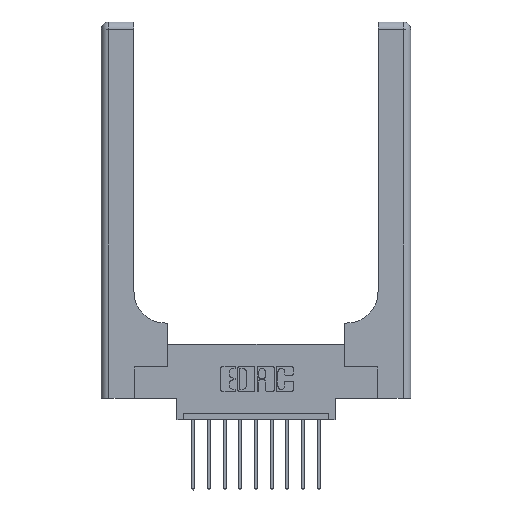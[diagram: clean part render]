
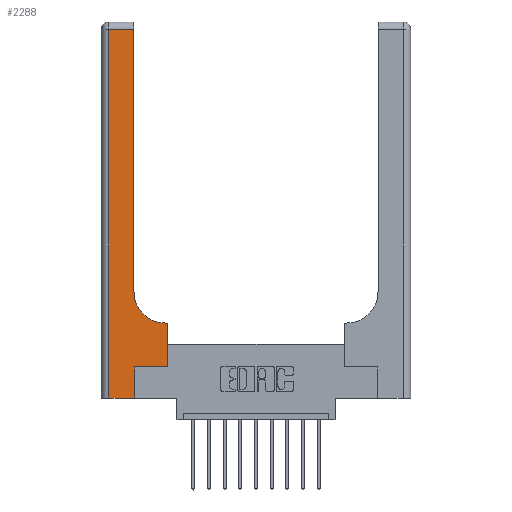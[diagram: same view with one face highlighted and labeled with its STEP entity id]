
A CAD part, top view. The second image highlights one B-rep face of the part: STEP entity #2288.
In plain terms, the highlighted planar face has unit normal (0, 0, 1).
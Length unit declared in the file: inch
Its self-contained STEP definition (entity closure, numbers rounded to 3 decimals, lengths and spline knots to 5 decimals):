
#54 = CARTESIAN_POINT ( 'NONE',  ( 0.51, 0.85, 0.37 ) ) ;
#245 = CARTESIAN_POINT ( 'NONE',  ( 0., 3., 0.37 ) ) ;
#322 = DIRECTION ( 'NONE',  ( 0., 1., 0. ) ) ;
#487 = VECTOR ( 'NONE', #4589, 39.37008 ) ;
#913 = ORIENTED_EDGE ( 'NONE', *, *, #4546, .T. ) ;
#1056 = VECTOR ( 'NONE', #8167, 39.37008 ) ;
#1525 = ORIENTED_EDGE ( 'NONE', *, *, #4933, .T. ) ;
#1647 = DIRECTION ( 'NONE',  ( 0., 1., 0. ) ) ;
#1715 = EDGE_LOOP ( 'NONE', ( #7475, #12008, #1525, #6539, #4272, #3460, #15296, #10799, #913 ) ) ;
#1851 = LINE ( 'NONE', #4492, #487 ) ;
#2288 = ADVANCED_FACE ( 'NONE', ( #4035 ), #2567, .F. ) ;
#2551 = EDGE_CURVE ( 'NONE', #13347, #2788, #5854, .T. ) ;
#2567 = PLANE ( 'NONE',  #7555 ) ;
#2635 = DIRECTION ( 'NONE',  ( 1., 0., 0. ) ) ;
#2788 = VERTEX_POINT ( 'NONE', #5135 ) ;
#3329 = EDGE_CURVE ( 'NONE', #9762, #10007, #15125, .T. ) ;
#3349 = CARTESIAN_POINT ( 'NONE',  ( 0.06, 0., 0.37 ) ) ;
#3460 = ORIENTED_EDGE ( 'NONE', *, *, #6564, .T. ) ;
#4035 = FACE_OUTER_BOUND ( 'NONE', #1715, .T. ) ;
#4132 = DIRECTION ( 'NONE',  ( -1., 0., 0. ) ) ;
#4255 = LINE ( 'NONE', #5275, #13698 ) ;
#4272 = ORIENTED_EDGE ( 'NONE', *, *, #3329, .T. ) ;
#4292 = VECTOR ( 'NONE', #4132, 39.37008 ) ;
#4322 = LINE ( 'NONE', #13469, #12302 ) ;
#4492 = CARTESIAN_POINT ( 'NONE',  ( 0.26, 0.6, 0.37 ) ) ;
#4546 = EDGE_CURVE ( 'NONE', #13623, #13347, #5232, .T. ) ;
#4589 = DIRECTION ( 'NONE',  ( -1., 0., 0. ) ) ;
#4761 = CARTESIAN_POINT ( 'NONE',  ( 0.26, 0.85, 0.37 ) ) ;
#4933 = EDGE_CURVE ( 'NONE', #6191, #13693, #4322, .T. ) ;
#5135 = CARTESIAN_POINT ( 'NONE',  ( 0.26, 2.94, 0.37 ) ) ;
#5178 = AXIS2_PLACEMENT_3D ( 'NONE', #54, #6262, #6154 ) ;
#5232 = CIRCLE ( 'NONE', #5178, 0.25 ) ;
#5275 = CARTESIAN_POINT ( 'NONE',  ( 0., 0., 0.37 ) ) ;
#5380 = LINE ( 'NONE', #6357, #12465 ) ;
#5854 = LINE ( 'NONE', #12187, #1056 ) ;
#6154 = DIRECTION ( 'NONE',  ( 1., 0., 0. ) ) ;
#6191 = VERTEX_POINT ( 'NONE', #14523 ) ;
#6262 = DIRECTION ( 'NONE',  ( 0., 0., -1. ) ) ;
#6357 = CARTESIAN_POINT ( 'NONE',  ( 0.265, 0.25, 0.37 ) ) ;
#6539 = ORIENTED_EDGE ( 'NONE', *, *, #7841, .T. ) ;
#6564 = EDGE_CURVE ( 'NONE', #10007, #10224, #5380, .T. ) ;
#7475 = ORIENTED_EDGE ( 'NONE', *, *, #2551, .T. ) ;
#7555 = AXIS2_PLACEMENT_3D ( 'NONE', #245, #13413, #12134 ) ;
#7587 = CARTESIAN_POINT ( 'NONE',  ( 0.528, 0.6, 0.37 ) ) ;
#7841 = EDGE_CURVE ( 'NONE', #13693, #9762, #4255, .T. ) ;
#8033 = CARTESIAN_POINT ( 'NONE',  ( 0.265, 0., 0.37 ) ) ;
#8057 = VECTOR ( 'NONE', #322, 39.37008 ) ;
#8167 = DIRECTION ( 'NONE',  ( 0., 1., 0. ) ) ;
#8651 = VECTOR ( 'NONE', #1647, 39.37008 ) ;
#8836 = DIRECTION ( 'NONE',  ( 0., -1., 0. ) ) ;
#9002 = CARTESIAN_POINT ( 'NONE',  ( 0.528, 0.25, 0.37 ) ) ;
#9458 = VERTEX_POINT ( 'NONE', #7587 ) ;
#9762 = VERTEX_POINT ( 'NONE', #8033 ) ;
#10007 = VERTEX_POINT ( 'NONE', #13125 ) ;
#10091 = EDGE_CURVE ( 'NONE', #10224, #9458, #12200, .T. ) ;
#10224 = VERTEX_POINT ( 'NONE', #9002 ) ;
#10799 = ORIENTED_EDGE ( 'NONE', *, *, #14190, .T. ) ;
#12008 = ORIENTED_EDGE ( 'NONE', *, *, #14170, .T. ) ;
#12134 = DIRECTION ( 'NONE',  ( -1., 0., 0. ) ) ;
#12187 = CARTESIAN_POINT ( 'NONE',  ( 0.26, 3., 0.37 ) ) ;
#12200 = LINE ( 'NONE', #12400, #8651 ) ;
#12302 = VECTOR ( 'NONE', #8836, 39.37008 ) ;
#12400 = CARTESIAN_POINT ( 'NONE',  ( 0.528, 0.25, 0.37 ) ) ;
#12465 = VECTOR ( 'NONE', #2635, 39.37008 ) ;
#12586 = CARTESIAN_POINT ( 'NONE',  ( 0., 2.94, 0.37 ) ) ;
#13053 = CARTESIAN_POINT ( 'NONE',  ( 0.51, 0.6, 0.37 ) ) ;
#13075 = CARTESIAN_POINT ( 'NONE',  ( 0.265, 0., 0.37 ) ) ;
#13125 = CARTESIAN_POINT ( 'NONE',  ( 0.265, 0.25, 0.37 ) ) ;
#13347 = VERTEX_POINT ( 'NONE', #4761 ) ;
#13386 = LINE ( 'NONE', #12586, #4292 ) ;
#13413 = DIRECTION ( 'NONE',  ( 0., 0., -1. ) ) ;
#13438 = DIRECTION ( 'NONE',  ( 1., 0., 0. ) ) ;
#13469 = CARTESIAN_POINT ( 'NONE',  ( 0.06, 3., 0.37 ) ) ;
#13623 = VERTEX_POINT ( 'NONE', #13053 ) ;
#13693 = VERTEX_POINT ( 'NONE', #3349 ) ;
#13698 = VECTOR ( 'NONE', #13438, 39.37008 ) ;
#14170 = EDGE_CURVE ( 'NONE', #2788, #6191, #13386, .T. ) ;
#14190 = EDGE_CURVE ( 'NONE', #9458, #13623, #1851, .T. ) ;
#14523 = CARTESIAN_POINT ( 'NONE',  ( 0.06, 2.94, 0.37 ) ) ;
#15125 = LINE ( 'NONE', #13075, #8057 ) ;
#15296 = ORIENTED_EDGE ( 'NONE', *, *, #10091, .T. ) ;
